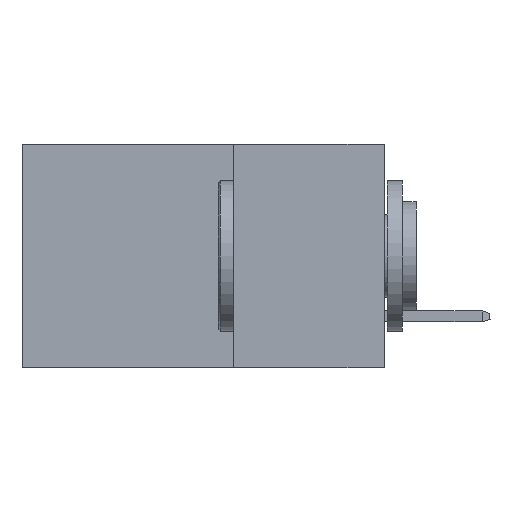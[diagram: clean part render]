
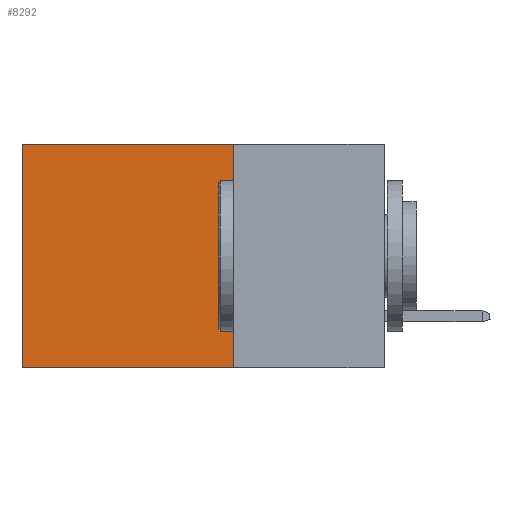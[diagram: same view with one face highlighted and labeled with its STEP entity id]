
A CAD part, left-side view. The second image highlights one B-rep face of the part: STEP entity #8292.
In plain terms, the highlighted planar face has unit normal (-1, 0, 0).
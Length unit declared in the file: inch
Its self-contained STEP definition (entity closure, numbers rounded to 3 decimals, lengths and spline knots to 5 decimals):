
#1498 = EDGE_CURVE ( 'NONE', #11777, #6216, #14085, .T. ) ;
#1570 = DIRECTION ( 'NONE',  ( 1., 0., 0. ) ) ;
#2041 = EDGE_CURVE ( 'NONE', #5036, #2748, #4172, .T. ) ;
#2103 = DIRECTION ( 'NONE',  ( 0., 1., 0. ) ) ;
#2745 = CARTESIAN_POINT ( 'NONE',  ( 0.2615, 0.6, 0. ) ) ;
#2748 = VERTEX_POINT ( 'NONE', #9445 ) ;
#3177 = CARTESIAN_POINT ( 'NONE',  ( 0.2615, 0.25, 0. ) ) ;
#3447 = EDGE_CURVE ( 'NONE', #11777, #5036, #10273, .T. ) ;
#4172 = LINE ( 'NONE', #7393, #9766 ) ;
#4193 = CARTESIAN_POINT ( 'NONE',  ( 0.2615, 0.25, -0.37 ) ) ;
#4298 = CARTESIAN_POINT ( 'NONE',  ( 0.2615, 0.25, -0.37 ) ) ;
#4989 = DIRECTION ( 'NONE',  ( 0., 0., -1. ) ) ;
#5036 = VERTEX_POINT ( 'NONE', #2745 ) ;
#5077 = CARTESIAN_POINT ( 'NONE',  ( 0.2615, 0.25, 0. ) ) ;
#5426 = EDGE_LOOP ( 'NONE', ( #8476, #7629, #9621, #8779 ) ) ;
#6216 = VERTEX_POINT ( 'NONE', #12891 ) ;
#7059 = CARTESIAN_POINT ( 'NONE',  ( 0.2615, 0.25, -0.37 ) ) ;
#7222 = VECTOR ( 'NONE', #11188, 39.37008 ) ;
#7393 = CARTESIAN_POINT ( 'NONE',  ( 0.2615, 0.6, -0.37 ) ) ;
#7629 = ORIENTED_EDGE ( 'NONE', *, *, #8572, .F. ) ;
#8292 = ADVANCED_FACE ( 'NONE', ( #9464 ), #8313, .F. ) ;
#8313 = PLANE ( 'NONE',  #11961 ) ;
#8476 = ORIENTED_EDGE ( 'NONE', *, *, #2041, .T. ) ;
#8572 = EDGE_CURVE ( 'NONE', #6216, #2748, #13396, .T. ) ;
#8779 = ORIENTED_EDGE ( 'NONE', *, *, #3447, .T. ) ;
#9445 = CARTESIAN_POINT ( 'NONE',  ( 0.2615, 0.6, -0.37 ) ) ;
#9464 = FACE_OUTER_BOUND ( 'NONE', #5426, .T. ) ;
#9621 = ORIENTED_EDGE ( 'NONE', *, *, #1498, .F. ) ;
#9766 = VECTOR ( 'NONE', #10827, 39.37008 ) ;
#9949 = VECTOR ( 'NONE', #14541, 39.37008 ) ;
#10273 = LINE ( 'NONE', #3177, #11528 ) ;
#10827 = DIRECTION ( 'NONE',  ( 0., 0., -1. ) ) ;
#11188 = DIRECTION ( 'NONE',  ( 0., 1., 0. ) ) ;
#11528 = VECTOR ( 'NONE', #2103, 39.37008 ) ;
#11777 = VERTEX_POINT ( 'NONE', #5077 ) ;
#11961 = AXIS2_PLACEMENT_3D ( 'NONE', #7059, #1570, #4989 ) ;
#12891 = CARTESIAN_POINT ( 'NONE',  ( 0.2615, 0.25, -0.37 ) ) ;
#13396 = LINE ( 'NONE', #4298, #7222 ) ;
#14085 = LINE ( 'NONE', #4193, #9949 ) ;
#14541 = DIRECTION ( 'NONE',  ( 0., 0., -1. ) ) ;
